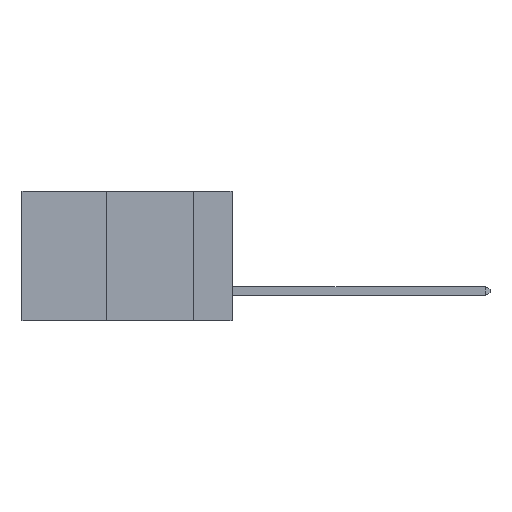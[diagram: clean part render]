
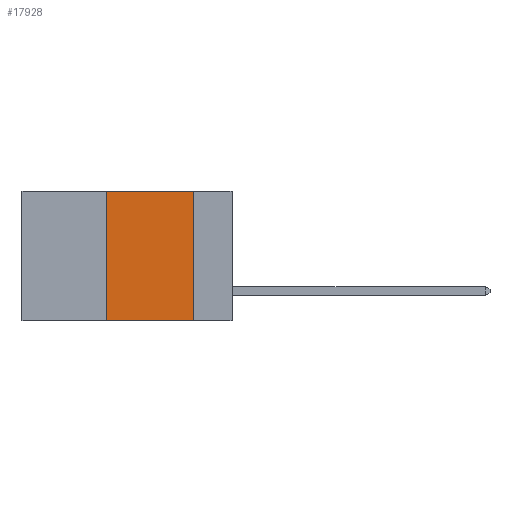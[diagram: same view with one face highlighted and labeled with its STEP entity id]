
A CAD part, left-side view. The second image highlights one B-rep face of the part: STEP entity #17928.
In plain terms, the highlighted planar face has unit normal (-1, 0, 0).
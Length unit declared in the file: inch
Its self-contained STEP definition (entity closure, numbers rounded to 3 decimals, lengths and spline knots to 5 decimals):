
#1066 = DIRECTION ( 'NONE',  ( 0., 0., -1. ) ) ;
#2402 = CARTESIAN_POINT ( 'NONE',  ( 0., 0.36, -0.37 ) ) ;
#2673 = ORIENTED_EDGE ( 'NONE', *, *, #30992, .F. ) ;
#3322 = VERTEX_POINT ( 'NONE', #8949 ) ;
#3327 = ORIENTED_EDGE ( 'NONE', *, *, #4949, .F. ) ;
#4462 = ORIENTED_EDGE ( 'NONE', *, *, #35108, .F. ) ;
#4949 = EDGE_CURVE ( 'NONE', #8059, #30524, #19085, .T. ) ;
#8059 = VERTEX_POINT ( 'NONE', #19591 ) ;
#8066 = LINE ( 'NONE', #19517, #31437 ) ;
#8949 = CARTESIAN_POINT ( 'NONE',  ( 0., 0.11, -0.37 ) ) ;
#9420 = DIRECTION ( 'NONE',  ( 0., 0., -1. ) ) ;
#9567 = FACE_OUTER_BOUND ( 'NONE', #14416, .T. ) ;
#10703 = CARTESIAN_POINT ( 'NONE',  ( 0., 0.6, -0.37 ) ) ;
#10739 = VERTEX_POINT ( 'NONE', #2402 ) ;
#11069 = DIRECTION ( 'NONE',  ( 0., -1., 0. ) ) ;
#13797 = DIRECTION ( 'NONE',  ( 0., -1., 0. ) ) ;
#14416 = EDGE_LOOP ( 'NONE', ( #2673, #3327, #4462, #24236 ) ) ;
#14474 = CARTESIAN_POINT ( 'NONE',  ( 0., 0.11, 0. ) ) ;
#17178 = VECTOR ( 'NONE', #11069, 39.37008 ) ;
#17308 = DIRECTION ( 'NONE',  ( 0., 0., 1. ) ) ;
#17626 = LINE ( 'NONE', #10703, #18597 ) ;
#17928 = ADVANCED_FACE ( 'NONE', ( #9567 ), #30610, .F. ) ;
#18597 = VECTOR ( 'NONE', #13797, 39.37008 ) ;
#19085 = LINE ( 'NONE', #20164, #17178 ) ;
#19517 = CARTESIAN_POINT ( 'NONE',  ( 0., 0.11, 0. ) ) ;
#19591 = CARTESIAN_POINT ( 'NONE',  ( 0., 0.36, 0. ) ) ;
#20164 = CARTESIAN_POINT ( 'NONE',  ( 0., 0.6, 0. ) ) ;
#21822 = VECTOR ( 'NONE', #17308, 39.37008 ) ;
#22784 = LINE ( 'NONE', #26488, #21822 ) ;
#24236 = ORIENTED_EDGE ( 'NONE', *, *, #33758, .T. ) ;
#24609 = CARTESIAN_POINT ( 'NONE',  ( 0., 0.6, 0. ) ) ;
#26488 = CARTESIAN_POINT ( 'NONE',  ( 0., 0.36, 0. ) ) ;
#27644 = DIRECTION ( 'NONE',  ( 1., 0., 0. ) ) ;
#30524 = VERTEX_POINT ( 'NONE', #14474 ) ;
#30610 = PLANE ( 'NONE',  #35980 ) ;
#30992 = EDGE_CURVE ( 'NONE', #30524, #3322, #8066, .T. ) ;
#31437 = VECTOR ( 'NONE', #1066, 39.37008 ) ;
#33758 = EDGE_CURVE ( 'NONE', #10739, #3322, #17626, .T. ) ;
#35108 = EDGE_CURVE ( 'NONE', #10739, #8059, #22784, .T. ) ;
#35980 = AXIS2_PLACEMENT_3D ( 'NONE', #24609, #27644, #9420 ) ;
